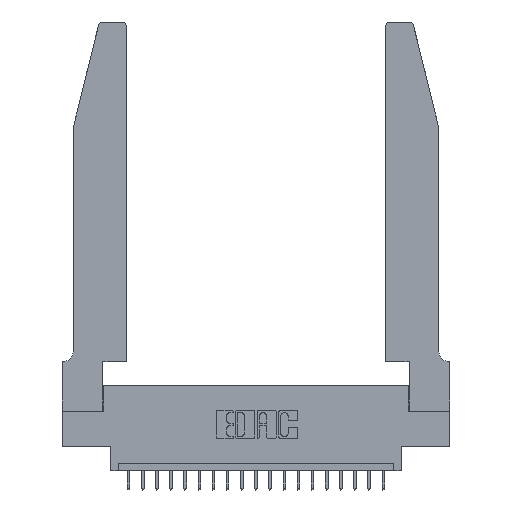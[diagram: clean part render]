
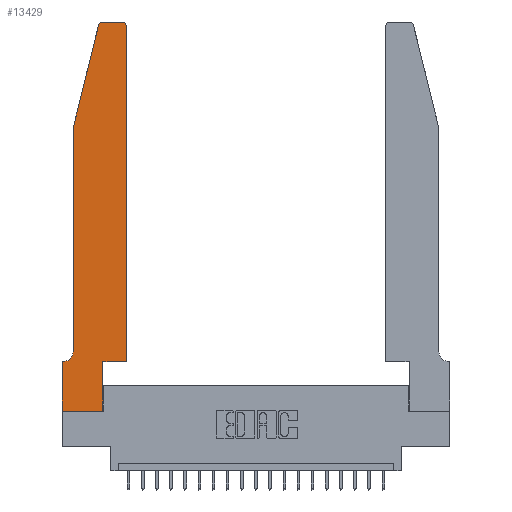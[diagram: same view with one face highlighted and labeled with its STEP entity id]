
A CAD part, top view. The second image highlights one B-rep face of the part: STEP entity #13429.
In plain terms, the highlighted planar face has unit normal (0, 0, 1).
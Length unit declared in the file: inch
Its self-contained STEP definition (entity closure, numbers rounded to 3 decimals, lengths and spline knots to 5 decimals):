
#332 = VERTEX_POINT ( 'NONE', #19429 ) ;
#390 = LINE ( 'NONE', #7278, #7991 ) ;
#990 = DIRECTION ( 'NONE',  ( 0., 0., 1. ) ) ;
#1015 = AXIS2_PLACEMENT_3D ( 'NONE', #18111, #990, #7870 ) ;
#1107 = CARTESIAN_POINT ( 'NONE',  ( 0.4505, 0.35, 0.37 ) ) ;
#1200 = CARTESIAN_POINT ( 'NONE',  ( 0.284, 2.75, 0.37 ) ) ;
#1328 = CARTESIAN_POINT ( 'NONE',  ( 0., 0., 0.37 ) ) ;
#1500 = ORIENTED_EDGE ( 'NONE', *, *, #18690, .T. ) ;
#1625 = EDGE_CURVE ( 'NONE', #20659, #10671, #2521, .T. ) ;
#1754 = CARTESIAN_POINT ( 'NONE',  ( 0.4505, 2.72, 0.37 ) ) ;
#1955 = VECTOR ( 'NONE', #20104, 39.37008 ) ;
#2270 = DIRECTION ( 'NONE',  ( -1., 0., 0. ) ) ;
#2462 = DIRECTION ( 'NONE',  ( 0., 0., 1. ) ) ;
#2521 = LINE ( 'NONE', #21775, #1955 ) ;
#2583 = VERTEX_POINT ( 'NONE', #7137 ) ;
#2657 = CIRCLE ( 'NONE', #9881, 0.03 ) ;
#2829 = CARTESIAN_POINT ( 'NONE',  ( 0.2865, 0.35, 0.37 ) ) ;
#3313 = DIRECTION ( 'NONE',  ( -0.239, -0.971, 0. ) ) ;
#3544 = LINE ( 'NONE', #13983, #22138 ) ;
#3577 = LINE ( 'NONE', #6859, #8445 ) ;
#3983 = LINE ( 'NONE', #14204, #20735 ) ;
#4171 = DIRECTION ( 'NONE',  ( 0., 0., 1. ) ) ;
#4326 = VECTOR ( 'NONE', #16822, 39.37008 ) ;
#4415 = AXIS2_PLACEMENT_3D ( 'NONE', #16202, #2462, #19723 ) ;
#5900 = DIRECTION ( 'NONE',  ( 0., 0., -1. ) ) ;
#6189 = LINE ( 'NONE', #13096, #14221 ) ;
#6304 = FACE_OUTER_BOUND ( 'NONE', #19118, .T. ) ;
#6350 = ORIENTED_EDGE ( 'NONE', *, *, #21090, .T. ) ;
#6721 = CARTESIAN_POINT ( 'NONE',  ( 0.2865, 0.35, 0.37 ) ) ;
#6727 = EDGE_CURVE ( 'NONE', #10671, #22066, #390, .T. ) ;
#6859 = CARTESIAN_POINT ( 'NONE',  ( 0.4505, 0.35, 0.37 ) ) ;
#7137 = CARTESIAN_POINT ( 'NONE',  ( 0.2865, 0., 0.37 ) ) ;
#7278 = CARTESIAN_POINT ( 'NONE',  ( 0., 0., 0.37 ) ) ;
#7681 = DIRECTION ( 'NONE',  ( 1., 0., 0. ) ) ;
#7870 = DIRECTION ( 'NONE',  ( 1., 0., 0. ) ) ;
#7991 = VECTOR ( 'NONE', #14218, 39.37008 ) ;
#8445 = VECTOR ( 'NONE', #19381, 39.37008 ) ;
#9361 = AXIS2_PLACEMENT_3D ( 'NONE', #14523, #5900, #2270 ) ;
#9400 = EDGE_CURVE ( 'NONE', #20294, #20323, #21438, .T. ) ;
#9554 = CARTESIAN_POINT ( 'NONE',  ( 0.0055, 0.35, 0.37 ) ) ;
#9817 = ORIENTED_EDGE ( 'NONE', *, *, #1625, .T. ) ;
#9850 = CARTESIAN_POINT ( 'NONE',  ( 0.4505, 0.35, 0.37 ) ) ;
#9881 = AXIS2_PLACEMENT_3D ( 'NONE', #21617, #4171, #7681 ) ;
#10113 = CARTESIAN_POINT ( 'NONE',  ( 0.25487, 2.72718, 0.37 ) ) ;
#10147 = VECTOR ( 'NONE', #15385, 39.37008 ) ;
#10215 = PLANE ( 'NONE',  #1015 ) ;
#10217 = ORIENTED_EDGE ( 'NONE', *, *, #20246, .T. ) ;
#10671 = VERTEX_POINT ( 'NONE', #13648 ) ;
#10760 = EDGE_CURVE ( 'NONE', #20323, #11265, #3544, .T. ) ;
#11184 = CIRCLE ( 'NONE', #9361, 0.07 ) ;
#11265 = VERTEX_POINT ( 'NONE', #17488 ) ;
#11958 = ORIENTED_EDGE ( 'NONE', *, *, #9400, .T. ) ;
#12101 = CARTESIAN_POINT ( 'NONE',  ( 0.4205, 2.75, 0.37 ) ) ;
#12615 = VERTEX_POINT ( 'NONE', #9850 ) ;
#12886 = ORIENTED_EDGE ( 'NONE', *, *, #14670, .T. ) ;
#12950 = ORIENTED_EDGE ( 'NONE', *, *, #21948, .T. ) ;
#13096 = CARTESIAN_POINT ( 'NONE',  ( 0.2605, 2.75, 0.37 ) ) ;
#13182 = CARTESIAN_POINT ( 'NONE',  ( 0., 0., 0.37 ) ) ;
#13429 = ADVANCED_FACE ( 'NONE', ( #6304 ), #10215, .T. ) ;
#13648 = CARTESIAN_POINT ( 'NONE',  ( 0., 0.35, 0.37 ) ) ;
#13863 = VECTOR ( 'NONE', #16692, 39.37008 ) ;
#13983 = CARTESIAN_POINT ( 'NONE',  ( 0.0755, 2., 0.37 ) ) ;
#14204 = CARTESIAN_POINT ( 'NONE',  ( 0.0755, 2., 0.37 ) ) ;
#14218 = DIRECTION ( 'NONE',  ( 0., -1., 0. ) ) ;
#14221 = VECTOR ( 'NONE', #20030, 39.37008 ) ;
#14264 = ORIENTED_EDGE ( 'NONE', *, *, #21184, .T. ) ;
#14523 = CARTESIAN_POINT ( 'NONE',  ( 0.0055, 0.42, 0.37 ) ) ;
#14670 = EDGE_CURVE ( 'NONE', #332, #20659, #11184, .T. ) ;
#15385 = DIRECTION ( 'NONE',  ( 0., 1., 0. ) ) ;
#15746 = ORIENTED_EDGE ( 'NONE', *, *, #6727, .T. ) ;
#16202 = CARTESIAN_POINT ( 'NONE',  ( 0.284, 2.72, 0.37 ) ) ;
#16475 = LINE ( 'NONE', #2829, #13863 ) ;
#16584 = DIRECTION ( 'NONE',  ( 0., -1., 0. ) ) ;
#16692 = DIRECTION ( 'NONE',  ( 0., 1., 0. ) ) ;
#16822 = DIRECTION ( 'NONE',  ( 1., 0., 0. ) ) ;
#17026 = ORIENTED_EDGE ( 'NONE', *, *, #22115, .T. ) ;
#17251 = ORIENTED_EDGE ( 'NONE', *, *, #17290, .T. ) ;
#17290 = EDGE_CURVE ( 'NONE', #22066, #2583, #20197, .T. ) ;
#17297 = ORIENTED_EDGE ( 'NONE', *, *, #10760, .T. ) ;
#17488 = CARTESIAN_POINT ( 'NONE',  ( 0.0755, 2., 0.37 ) ) ;
#18111 = CARTESIAN_POINT ( 'NONE',  ( 0., 0.35, 0.37 ) ) ;
#18483 = VERTEX_POINT ( 'NONE', #12101 ) ;
#18690 = EDGE_CURVE ( 'NONE', #12615, #20046, #22270, .T. ) ;
#19118 = EDGE_LOOP ( 'NONE', ( #10217, #11958, #17297, #6350, #12886, #9817, #15746, #17251, #14264, #17026, #1500, #12950 ) ) ;
#19289 = VERTEX_POINT ( 'NONE', #6721 ) ;
#19381 = DIRECTION ( 'NONE',  ( 1., 0., 0. ) ) ;
#19429 = CARTESIAN_POINT ( 'NONE',  ( 0.0755, 0.42, 0.37 ) ) ;
#19723 = DIRECTION ( 'NONE',  ( 1., 0., 0. ) ) ;
#20030 = DIRECTION ( 'NONE',  ( -1., 0., 0. ) ) ;
#20046 = VERTEX_POINT ( 'NONE', #1754 ) ;
#20104 = DIRECTION ( 'NONE',  ( -1., 0., 0. ) ) ;
#20197 = LINE ( 'NONE', #13182, #4326 ) ;
#20246 = EDGE_CURVE ( 'NONE', #18483, #20294, #6189, .T. ) ;
#20294 = VERTEX_POINT ( 'NONE', #1200 ) ;
#20323 = VERTEX_POINT ( 'NONE', #10113 ) ;
#20659 = VERTEX_POINT ( 'NONE', #9554 ) ;
#20735 = VECTOR ( 'NONE', #16584, 39.37008 ) ;
#21090 = EDGE_CURVE ( 'NONE', #11265, #332, #3983, .T. ) ;
#21184 = EDGE_CURVE ( 'NONE', #2583, #19289, #16475, .T. ) ;
#21438 = CIRCLE ( 'NONE', #4415, 0.03 ) ;
#21617 = CARTESIAN_POINT ( 'NONE',  ( 0.4205, 2.72, 0.37 ) ) ;
#21775 = CARTESIAN_POINT ( 'NONE',  ( 0.0755, 0.35, 0.37 ) ) ;
#21948 = EDGE_CURVE ( 'NONE', #20046, #18483, #2657, .T. ) ;
#22066 = VERTEX_POINT ( 'NONE', #1328 ) ;
#22115 = EDGE_CURVE ( 'NONE', #19289, #12615, #3577, .T. ) ;
#22138 = VECTOR ( 'NONE', #3313, 39.37008 ) ;
#22270 = LINE ( 'NONE', #1107, #10147 ) ;
